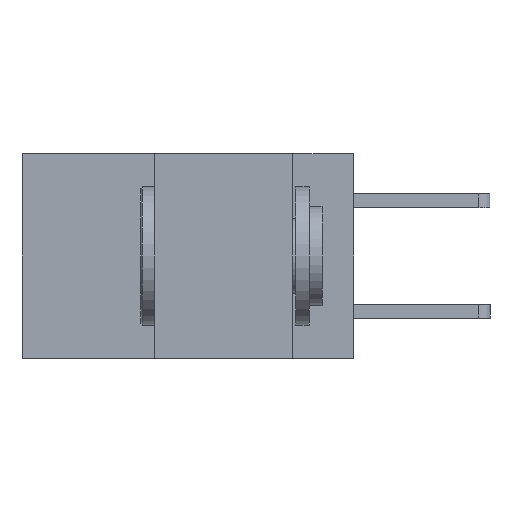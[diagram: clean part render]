
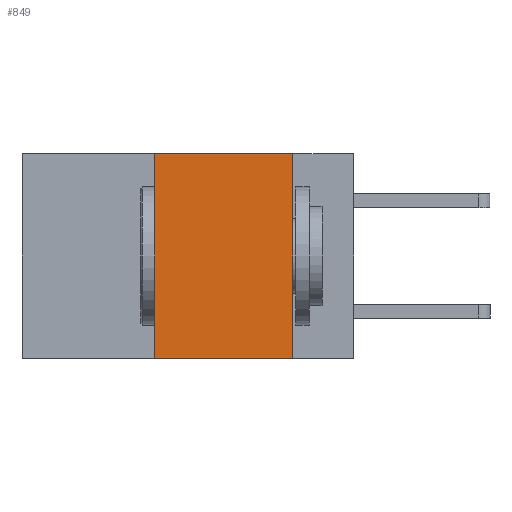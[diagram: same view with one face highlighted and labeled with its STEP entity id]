
A CAD part, left-side view. The second image highlights one B-rep face of the part: STEP entity #849.
In plain terms, the highlighted planar face has unit normal (-1, 0, 0).
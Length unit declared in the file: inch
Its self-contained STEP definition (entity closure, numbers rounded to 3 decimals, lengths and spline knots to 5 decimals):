
#43 = EDGE_CURVE ( 'NONE', #8003, #5007, #1649, .T. ) ;
#213 = EDGE_CURVE ( 'NONE', #8003, #2805, #5230, .T. ) ;
#475 = VECTOR ( 'NONE', #6099, 39.37008 ) ;
#729 = VECTOR ( 'NONE', #4349, 39.37008 ) ;
#813 = CARTESIAN_POINT ( 'NONE',  ( 0., 0.6, 0. ) ) ;
#849 = ADVANCED_FACE ( 'NONE', ( #7512 ), #6121, .F. ) ;
#994 = LINE ( 'NONE', #2515, #475 ) ;
#1507 = EDGE_CURVE ( 'NONE', #8042, #2805, #4354, .T. ) ;
#1649 = LINE ( 'NONE', #2951, #4778 ) ;
#2173 = DIRECTION ( 'NONE',  ( 0., 0., -1. ) ) ;
#2211 = EDGE_LOOP ( 'NONE', ( #8364, #4731, #3173, #4061 ) ) ;
#2438 = DIRECTION ( 'NONE',  ( 1., 0., 0. ) ) ;
#2515 = CARTESIAN_POINT ( 'NONE',  ( 0., 0.6, 0. ) ) ;
#2805 = VERTEX_POINT ( 'NONE', #6911 ) ;
#2841 = CARTESIAN_POINT ( 'NONE',  ( 0., 0.36, -0.37 ) ) ;
#2951 = CARTESIAN_POINT ( 'NONE',  ( 0., 0.36, 0. ) ) ;
#3023 = CARTESIAN_POINT ( 'NONE',  ( 0., 0.6, -0.37 ) ) ;
#3173 = ORIENTED_EDGE ( 'NONE', *, *, #43, .F. ) ;
#4061 = ORIENTED_EDGE ( 'NONE', *, *, #213, .T. ) ;
#4349 = DIRECTION ( 'NONE',  ( 0., -1., 0. ) ) ;
#4354 = LINE ( 'NONE', #5856, #5742 ) ;
#4633 = AXIS2_PLACEMENT_3D ( 'NONE', #813, #2438, #5543 ) ;
#4731 = ORIENTED_EDGE ( 'NONE', *, *, #8488, .F. ) ;
#4778 = VECTOR ( 'NONE', #6693, 39.37008 ) ;
#5007 = VERTEX_POINT ( 'NONE', #7882 ) ;
#5230 = LINE ( 'NONE', #3023, #729 ) ;
#5285 = CARTESIAN_POINT ( 'NONE',  ( 0., 0.11, 0. ) ) ;
#5543 = DIRECTION ( 'NONE',  ( 0., 0., -1. ) ) ;
#5742 = VECTOR ( 'NONE', #2173, 39.37008 ) ;
#5856 = CARTESIAN_POINT ( 'NONE',  ( 0., 0.11, 0. ) ) ;
#6099 = DIRECTION ( 'NONE',  ( 0., -1., 0. ) ) ;
#6121 = PLANE ( 'NONE',  #4633 ) ;
#6693 = DIRECTION ( 'NONE',  ( 0., 0., 1. ) ) ;
#6911 = CARTESIAN_POINT ( 'NONE',  ( 0., 0.11, -0.37 ) ) ;
#7512 = FACE_OUTER_BOUND ( 'NONE', #2211, .T. ) ;
#7882 = CARTESIAN_POINT ( 'NONE',  ( 0., 0.36, 0. ) ) ;
#8003 = VERTEX_POINT ( 'NONE', #2841 ) ;
#8042 = VERTEX_POINT ( 'NONE', #5285 ) ;
#8364 = ORIENTED_EDGE ( 'NONE', *, *, #1507, .F. ) ;
#8488 = EDGE_CURVE ( 'NONE', #5007, #8042, #994, .T. ) ;
